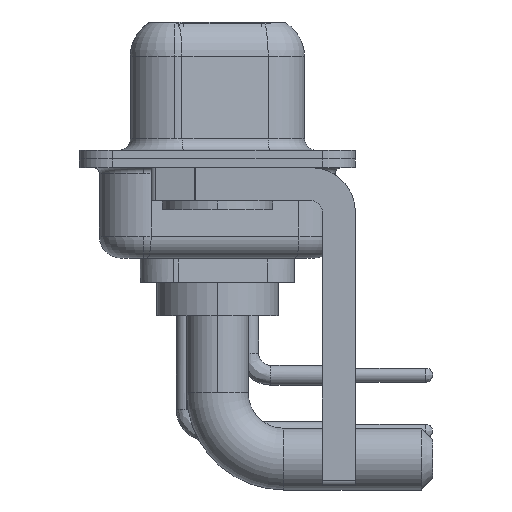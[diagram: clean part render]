
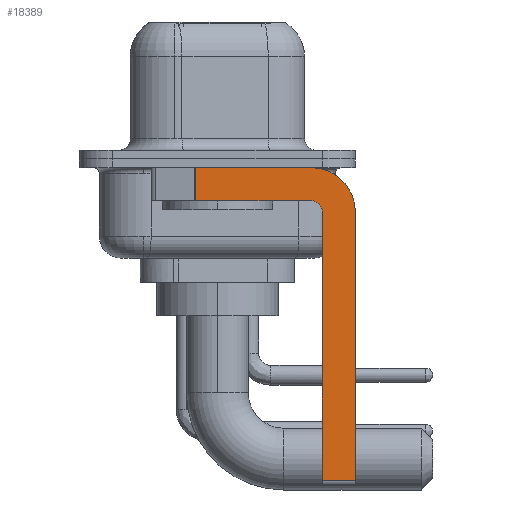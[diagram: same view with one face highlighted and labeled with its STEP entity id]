
A CAD part, left-side view. The second image highlights one B-rep face of the part: STEP entity #18389.
In plain terms, the highlighted planar face has unit normal (-1, 0, 0).
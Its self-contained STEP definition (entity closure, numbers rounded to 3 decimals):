
#350 = LINE ( 'NONE', #1655, #8714 ) ;
#1274 = CARTESIAN_POINT ( 'NONE',  ( -2.9, -4.25, -2.4 ) ) ;
#1311 = CARTESIAN_POINT ( 'NONE',  ( -2.9, 0.978, -1.9 ) ) ;
#1336 = CARTESIAN_POINT ( 'NONE',  ( -2.9, -4.25, -14.55 ) ) ;
#1587 = CARTESIAN_POINT ( 'NONE',  ( -2.9, -4.75, -2.4 ) ) ;
#1655 = CARTESIAN_POINT ( 'NONE',  ( -2.9, 3., -0.4 ) ) ;
#1876 = ORIENTED_EDGE ( 'NONE', *, *, #15359, .F. ) ;
#2448 = AXIS2_PLACEMENT_3D ( 'NONE', #1274, #2696, #2895 ) ;
#2602 = CARTESIAN_POINT ( 'NONE',  ( -2.9, -4.25, -2.4 ) ) ;
#2696 = DIRECTION ( 'NONE',  ( 1., 0., 0. ) ) ;
#2809 = VECTOR ( 'NONE', #15589, 1000. ) ;
#2895 = DIRECTION ( 'NONE',  ( 0., 0., -1. ) ) ;
#3166 = CARTESIAN_POINT ( 'NONE',  ( -2.9, -4.25, -0.4 ) ) ;
#3168 = ORIENTED_EDGE ( 'NONE', *, *, #13283, .F. ) ;
#3693 = EDGE_CURVE ( 'NONE', #17509, #8041, #19510, .T. ) ;
#3803 = CARTESIAN_POINT ( 'NONE',  ( -2.9, -4.75, -14.55 ) ) ;
#4101 = DIRECTION ( 'NONE',  ( 0., 0., 1. ) ) ;
#4467 = LINE ( 'NONE', #1336, #8174 ) ;
#5543 = VECTOR ( 'NONE', #17922, 1000. ) ;
#5573 = DIRECTION ( 'NONE',  ( 0., 0., 1. ) ) ;
#5627 = DIRECTION ( 'NONE',  ( 0., 0., -1. ) ) ;
#5979 = VERTEX_POINT ( 'NONE', #10249 ) ;
#6114 = EDGE_CURVE ( 'NONE', #13840, #10291, #350, .T. ) ;
#6958 = ORIENTED_EDGE ( 'NONE', *, *, #8708, .F. ) ;
#7129 = AXIS2_PLACEMENT_3D ( 'NONE', #2602, #13446, #5627 ) ;
#7557 = CARTESIAN_POINT ( 'NONE',  ( -2.9, 0.978, -1.9 ) ) ;
#7603 = DIRECTION ( 'NONE',  ( 0., -1., 0. ) ) ;
#7647 = CARTESIAN_POINT ( 'NONE',  ( -2.9, -6.25, -14.55 ) ) ;
#7862 = EDGE_CURVE ( 'NONE', #10291, #17050, #10328, .T. ) ;
#7909 = VERTEX_POINT ( 'NONE', #7647 ) ;
#8041 = VERTEX_POINT ( 'NONE', #1587 ) ;
#8174 = VECTOR ( 'NONE', #7603, 1000. ) ;
#8450 = AXIS2_PLACEMENT_3D ( 'NONE', #11715, #17843, #4101 ) ;
#8708 = EDGE_CURVE ( 'NONE', #5979, #13485, #17623, .T. ) ;
#8714 = VECTOR ( 'NONE', #12508, 1000. ) ;
#9480 = LINE ( 'NONE', #9671, #2809 ) ;
#9671 = CARTESIAN_POINT ( 'NONE',  ( -2.9, -6.25, -2.4 ) ) ;
#10249 = CARTESIAN_POINT ( 'NONE',  ( -2.9, -4.25, -1.9 ) ) ;
#10291 = VERTEX_POINT ( 'NONE', #3166 ) ;
#10325 = EDGE_CURVE ( 'NONE', #17509, #7909, #4467, .T. ) ;
#10328 = CIRCLE ( 'NONE', #7129, 2. ) ;
#10865 = DIRECTION ( 'NONE',  ( 0., 0., -1. ) ) ;
#11195 = EDGE_CURVE ( 'NONE', #13840, #13485, #12064, .T. ) ;
#11546 = VECTOR ( 'NONE', #5573, 1000. ) ;
#11649 = CARTESIAN_POINT ( 'NONE',  ( -2.9, -6.25, -2.4 ) ) ;
#11715 = CARTESIAN_POINT ( 'NONE',  ( -2.9, -4.25, -2.4 ) ) ;
#12064 = LINE ( 'NONE', #1311, #16835 ) ;
#12128 = PLANE ( 'NONE',  #2448 ) ;
#12508 = DIRECTION ( 'NONE',  ( 0., -1., 0. ) ) ;
#12968 = ORIENTED_EDGE ( 'NONE', *, *, #6114, .F. ) ;
#12980 = ORIENTED_EDGE ( 'NONE', *, *, #10325, .T. ) ;
#13283 = EDGE_CURVE ( 'NONE', #17050, #7909, #9480, .T. ) ;
#13413 = EDGE_LOOP ( 'NONE', ( #12968, #15963, #6958, #1876, #18800, #12980, #3168, #15418 ) ) ;
#13446 = DIRECTION ( 'NONE',  ( 1., 0., 0. ) ) ;
#13485 = VERTEX_POINT ( 'NONE', #7557 ) ;
#13840 = VERTEX_POINT ( 'NONE', #19248 ) ;
#15359 = EDGE_CURVE ( 'NONE', #8041, #5979, #16434, .T. ) ;
#15418 = ORIENTED_EDGE ( 'NONE', *, *, #7862, .F. ) ;
#15589 = DIRECTION ( 'NONE',  ( 0., 0., -1. ) ) ;
#15963 = ORIENTED_EDGE ( 'NONE', *, *, #11195, .T. ) ;
#16434 = CIRCLE ( 'NONE', #8450, 0.5 ) ;
#16832 = FACE_OUTER_BOUND ( 'NONE', #13413, .T. ) ;
#16835 = VECTOR ( 'NONE', #10865, 1000. ) ;
#17050 = VERTEX_POINT ( 'NONE', #11649 ) ;
#17509 = VERTEX_POINT ( 'NONE', #3803 ) ;
#17623 = LINE ( 'NONE', #17818, #5543 ) ;
#17818 = CARTESIAN_POINT ( 'NONE',  ( -2.9, -4.25, -1.9 ) ) ;
#17843 = DIRECTION ( 'NONE',  ( -1., 0., 0. ) ) ;
#17922 = DIRECTION ( 'NONE',  ( 0., 1., 0. ) ) ;
#18117 = CARTESIAN_POINT ( 'NONE',  ( -2.9, -4.75, -14.8 ) ) ;
#18389 = ADVANCED_FACE ( 'NONE', ( #16832 ), #12128, .F. ) ;
#18800 = ORIENTED_EDGE ( 'NONE', *, *, #3693, .F. ) ;
#19248 = CARTESIAN_POINT ( 'NONE',  ( -2.9, 0.978, -0.4 ) ) ;
#19510 = LINE ( 'NONE', #18117, #11546 ) ;
